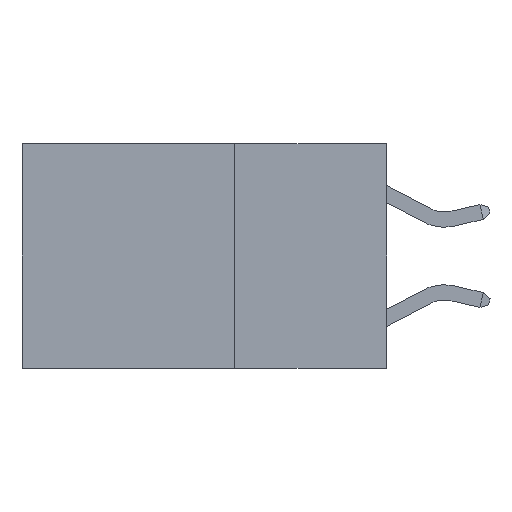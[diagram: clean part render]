
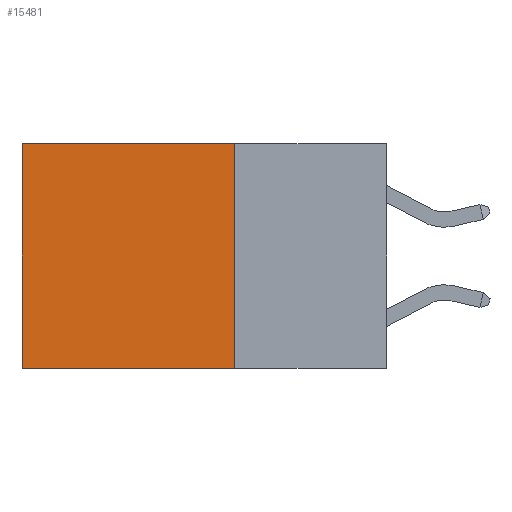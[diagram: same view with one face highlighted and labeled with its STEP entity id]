
A CAD part, left-side view. The second image highlights one B-rep face of the part: STEP entity #15481.
In plain terms, the highlighted planar face has unit normal (-1, 0, 0).
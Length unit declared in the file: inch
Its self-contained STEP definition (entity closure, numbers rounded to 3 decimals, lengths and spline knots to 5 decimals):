
#3 = ORIENTED_EDGE ( 'NONE', *, *, #16684, .F. ) ;
#353 = FACE_OUTER_BOUND ( 'NONE', #4772, .T. ) ;
#796 = LINE ( 'NONE', #8460, #17239 ) ;
#1241 = VERTEX_POINT ( 'NONE', #21328 ) ;
#1788 = VECTOR ( 'NONE', #8892, 39.37008 ) ;
#2371 = CARTESIAN_POINT ( 'NONE',  ( 0.2625, 0.6, 0. ) ) ;
#3347 = CARTESIAN_POINT ( 'NONE',  ( 0.2625, 0.25, 0. ) ) ;
#3578 = CARTESIAN_POINT ( 'NONE',  ( 0.2625, 0.25, 0. ) ) ;
#3788 = CARTESIAN_POINT ( 'NONE',  ( 0.2625, 0.25, 0. ) ) ;
#4772 = EDGE_LOOP ( 'NONE', ( #25109, #3, #20483, #13993 ) ) ;
#4853 = VERTEX_POINT ( 'NONE', #15261 ) ;
#5387 = VERTEX_POINT ( 'NONE', #19443 ) ;
#5965 = DIRECTION ( 'NONE',  ( 0., 0., -1. ) ) ;
#8460 = CARTESIAN_POINT ( 'NONE',  ( 0.2625, 0.25, 0. ) ) ;
#8658 = EDGE_CURVE ( 'NONE', #20654, #5387, #26732, .T. ) ;
#8892 = DIRECTION ( 'NONE',  ( 0., 0., -1. ) ) ;
#8904 = LINE ( 'NONE', #2371, #1788 ) ;
#9041 = AXIS2_PLACEMENT_3D ( 'NONE', #3788, #18732, #5965 ) ;
#9713 = VECTOR ( 'NONE', #9999, 39.37008 ) ;
#9999 = DIRECTION ( 'NONE',  ( 0., 1., 0. ) ) ;
#13993 = ORIENTED_EDGE ( 'NONE', *, *, #25372, .T. ) ;
#14452 = EDGE_CURVE ( 'NONE', #1241, #4853, #8904, .T. ) ;
#15261 = CARTESIAN_POINT ( 'NONE',  ( 0.2625, 0.6, -0.37 ) ) ;
#15481 = ADVANCED_FACE ( 'NONE', ( #353 ), #25094, .F. ) ;
#16123 = DIRECTION ( 'NONE',  ( 0., 0., -1. ) ) ;
#16322 = CARTESIAN_POINT ( 'NONE',  ( 0.2625, 0.25, -0.37 ) ) ;
#16684 = EDGE_CURVE ( 'NONE', #5387, #4853, #26771, .T. ) ;
#17239 = VECTOR ( 'NONE', #21227, 39.37008 ) ;
#18732 = DIRECTION ( 'NONE',  ( 1., 0., 0. ) ) ;
#19443 = CARTESIAN_POINT ( 'NONE',  ( 0.2625, 0.25, -0.37 ) ) ;
#20376 = VECTOR ( 'NONE', #16123, 39.37008 ) ;
#20483 = ORIENTED_EDGE ( 'NONE', *, *, #8658, .F. ) ;
#20654 = VERTEX_POINT ( 'NONE', #3578 ) ;
#21227 = DIRECTION ( 'NONE',  ( 0., 1., 0. ) ) ;
#21328 = CARTESIAN_POINT ( 'NONE',  ( 0.2625, 0.6, 0. ) ) ;
#25094 = PLANE ( 'NONE',  #9041 ) ;
#25109 = ORIENTED_EDGE ( 'NONE', *, *, #14452, .T. ) ;
#25372 = EDGE_CURVE ( 'NONE', #20654, #1241, #796, .T. ) ;
#26732 = LINE ( 'NONE', #3347, #20376 ) ;
#26771 = LINE ( 'NONE', #16322, #9713 ) ;
